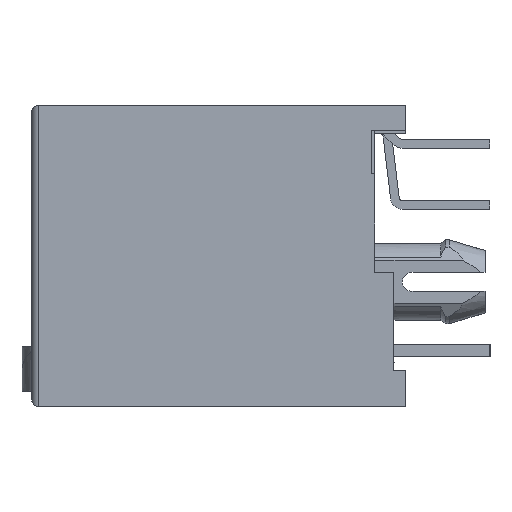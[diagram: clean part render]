
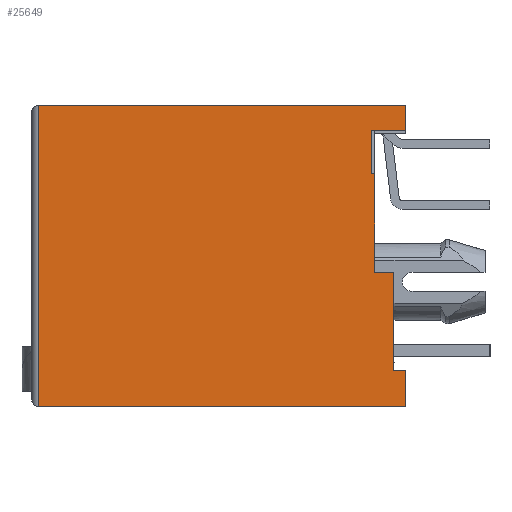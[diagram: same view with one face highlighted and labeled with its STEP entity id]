
A CAD part, left-side view. The second image highlights one B-rep face of the part: STEP entity #25649.
In plain terms, the highlighted planar face has unit normal (-1, 0, 0).
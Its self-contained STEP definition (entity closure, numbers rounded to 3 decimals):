
#753 = CARTESIAN_POINT ( 'NONE',  ( -31.5, -6.35, 5.25 ) ) ;
#794 = B_SPLINE_CURVE_WITH_KNOTS ( 'NONE', 3,
 ( #58635, #41597, #31575, #52711 ),
 .UNSPECIFIED., .F., .F.,
 ( 4, 4 ),
 ( 0., 1. ),
 .UNSPECIFIED. ) ;
#1105 = CARTESIAN_POINT ( 'NONE',  ( -31.5, -7.3, -4.75 ) ) ;
#1653 = FACE_OUTER_BOUND ( 'NONE', #20320, .T. ) ;
#1766 = PLANE ( 'NONE',  #33108 ) ;
#1990 = ORIENTED_EDGE ( 'NONE', *, *, #2348, .F. ) ;
#2241 = CARTESIAN_POINT ( 'NONE',  ( -31.5, 7.806, -6.501 ) ) ;
#2348 = EDGE_CURVE ( 'NONE', #6272, #35705, #45475, .T. ) ;
#3171 = CARTESIAN_POINT ( 'NONE',  ( -31.5, -7.8, 5.95 ) ) ;
#3484 = CARTESIAN_POINT ( 'NONE',  ( -31.5, 7.5, -6.25 ) ) ;
#4537 = CARTESIAN_POINT ( 'NONE',  ( -31.5, -7.317, 5.25 ) ) ;
#4811 = CARTESIAN_POINT ( 'NONE',  ( -31.5, -7.3, -0.65 ) ) ;
#5822 = VERTEX_POINT ( 'NONE', #54290 ) ;
#5999 = CARTESIAN_POINT ( 'NONE',  ( -31.5, -7.3, -0.65 ) ) ;
#6272 = VERTEX_POINT ( 'NONE', #4811 ) ;
#6521 = CARTESIAN_POINT ( 'NONE',  ( -31.5, -7.8, -4.75 ) ) ;
#6751 = CARTESIAN_POINT ( 'NONE',  ( -31.5, -7.633, -4.75 ) ) ;
#7756 = EDGE_CURVE ( 'NONE', #69774, #23498, #36335, .T. ) ;
#8412 = EDGE_CURVE ( 'NONE', #5822, #59870, #36721, .T. ) ;
#8703 = CARTESIAN_POINT ( 'NONE',  ( -31.5, -6.4, 3.45 ) ) ;
#8846 = CARTESIAN_POINT ( 'NONE',  ( -31.5, -7.8, 5.25 ) ) ;
#9797 = EDGE_CURVE ( 'NONE', #43913, #19857, #70163, .T. ) ;
#10039 = CARTESIAN_POINT ( 'NONE',  ( -31.5, -7.8, -6.25 ) ) ;
#10140 = CARTESIAN_POINT ( 'NONE',  ( -31.5, -7.3, -0.65 ) ) ;
#12160 = CARTESIAN_POINT ( 'NONE',  ( -31.5, -7.3, -4.75 ) ) ;
#13658 = CARTESIAN_POINT ( 'NONE',  ( -31.5, -6.5, 3.45 ) ) ;
#14798 = VERTEX_POINT ( 'NONE', #19851 ) ;
#15674 = EDGE_CURVE ( 'NONE', #24459, #54209, #63186, .T. ) ;
#16421 = B_SPLINE_CURVE_WITH_KNOTS ( 'NONE', 3,
 ( #46222, #8703, #41508, #13658 ),
 .UNSPECIFIED., .F., .F.,
 ( 4, 4 ),
 ( 0., 1. ),
 .UNSPECIFIED. ) ;
#17293 = CARTESIAN_POINT ( 'NONE',  ( -31.5, 2.4, 6.3 ) ) ;
#18165 = CARTESIAN_POINT ( 'NONE',  ( -31.5, -7.8, 5.25 ) ) ;
#18745 = B_SPLINE_CURVE_WITH_KNOTS ( 'NONE', 3,
 ( #1105, #39566, #6751, #6521 ),
 .UNSPECIFIED., .F., .F.,
 ( 4, 4 ),
 ( 0., 1. ),
 .UNSPECIFIED. ) ;
#19851 = CARTESIAN_POINT ( 'NONE',  ( -31.5, -6.5, 3.45 ) ) ;
#19857 = VERTEX_POINT ( 'NONE', #50741 ) ;
#20320 = EDGE_LOOP ( 'NONE', ( #28924, #63908, #1990, #67134, #37770, #33921, #66121, #42720, #31346, #48273, #62933, #54552 ) ) ;
#21495 = EDGE_CURVE ( 'NONE', #19857, #14798, #16421, .T. ) ;
#22341 = EDGE_CURVE ( 'NONE', #54209, #23498, #27360, .T. ) ;
#23498 = VERTEX_POINT ( 'NONE', #67031 ) ;
#23927 = CARTESIAN_POINT ( 'NONE',  ( -31.5, -7.8, -4.75 ) ) ;
#24459 = VERTEX_POINT ( 'NONE', #23927 ) ;
#25649 = ADVANCED_FACE ( 'NONE', ( #1653 ), #1766, .F. ) ;
#25745 = CARTESIAN_POINT ( 'NONE',  ( -31.5, -7.8, -4.75 ) ) ;
#27360 = B_SPLINE_CURVE_WITH_KNOTS ( 'NONE', 3,
 ( #43266, #48709, #38516, #59850 ),
 .UNSPECIFIED., .F., .F.,
 ( 4, 4 ),
 ( 0., 1. ),
 .UNSPECIFIED. ) ;
#28924 = ORIENTED_EDGE ( 'NONE', *, *, #15674, .F. ) ;
#29045 = DIRECTION ( 'NONE',  ( 1., 0., 0. ) ) ;
#29296 = CARTESIAN_POINT ( 'NONE',  ( -31.5, -6.35, 4.05 ) ) ;
#30078 = CARTESIAN_POINT ( 'NONE',  ( -31.5, 7.5, 6.3 ) ) ;
#30939 = B_SPLINE_CURVE_WITH_KNOTS ( 'NONE', 3,
 ( #36412, #4537, #47968, #52745 ),
 .UNSPECIFIED., .F., .F.,
 ( 4, 4 ),
 ( 0., 1. ),
 .UNSPECIFIED. ) ;
#31346 = ORIENTED_EDGE ( 'NONE', *, *, #8412, .F. ) ;
#31424 = EDGE_CURVE ( 'NONE', #35705, #24459, #18745, .T. ) ;
#31575 = CARTESIAN_POINT ( 'NONE',  ( -31.5, -6.5, 0.717 ) ) ;
#33108 = AXIS2_PLACEMENT_3D ( 'NONE', #2241, #29045, #45415 ) ;
#33334 = CARTESIAN_POINT ( 'NONE',  ( -31.5, 7.5, 6.3 ) ) ;
#33423 = CARTESIAN_POINT ( 'NONE',  ( -31.5, -2.7, 6.3 ) ) ;
#33921 = ORIENTED_EDGE ( 'NONE', *, *, #21495, .F. ) ;
#34442 = B_SPLINE_CURVE_WITH_KNOTS ( 'NONE', 3,
 ( #47892, #37257, #58598, #10140 ),
 .UNSPECIFIED., .F., .F.,
 ( 4, 4 ),
 ( 0., 1. ),
 .UNSPECIFIED. ) ;
#35705 = VERTEX_POINT ( 'NONE', #12160 ) ;
#36335 = B_SPLINE_CURVE_WITH_KNOTS ( 'NONE', 3,
 ( #30078, #51194, #68269, #3484 ),
 .UNSPECIFIED., .F., .F.,
 ( 4, 4 ),
 ( 0., 1. ),
 .UNSPECIFIED. ) ;
#36412 = CARTESIAN_POINT ( 'NONE',  ( -31.5, -7.8, 5.25 ) ) ;
#36721 = B_SPLINE_CURVE_WITH_KNOTS ( 'NONE', 3,
 ( #62959, #3171, #52290, #8846 ),
 .UNSPECIFIED., .F., .F.,
 ( 4, 4 ),
 ( 0., 1. ),
 .UNSPECIFIED. ) ;
#37158 = CARTESIAN_POINT ( 'NONE',  ( -31.5, -7.8, -5.25 ) ) ;
#37257 = CARTESIAN_POINT ( 'NONE',  ( -31.5, -6.767, -0.65 ) ) ;
#37770 = ORIENTED_EDGE ( 'NONE', *, *, #45168, .F. ) ;
#38516 = CARTESIAN_POINT ( 'NONE',  ( -31.5, 2.4, -6.25 ) ) ;
#38568 = CARTESIAN_POINT ( 'NONE',  ( -31.5, -7.3, -4.75 ) ) ;
#39542 = CARTESIAN_POINT ( 'NONE',  ( -31.5, -6.35, 5.25 ) ) ;
#39566 = CARTESIAN_POINT ( 'NONE',  ( -31.5, -7.467, -4.75 ) ) ;
#40373 = CARTESIAN_POINT ( 'NONE',  ( -31.5, -7.8, -6.25 ) ) ;
#41508 = CARTESIAN_POINT ( 'NONE',  ( -31.5, -6.45, 3.45 ) ) ;
#41597 = CARTESIAN_POINT ( 'NONE',  ( -31.5, -6.5, 2.083 ) ) ;
#42174 = EDGE_CURVE ( 'NONE', #59870, #43913, #30939, .T. ) ;
#42597 = CARTESIAN_POINT ( 'NONE',  ( -31.5, -7.8, -5.75 ) ) ;
#42720 = ORIENTED_EDGE ( 'NONE', *, *, #42174, .F. ) ;
#43266 = CARTESIAN_POINT ( 'NONE',  ( -31.5, -7.8, -6.25 ) ) ;
#43913 = VERTEX_POINT ( 'NONE', #753 ) ;
#44025 = CARTESIAN_POINT ( 'NONE',  ( -31.5, -7.3, -2.017 ) ) ;
#45168 = EDGE_CURVE ( 'NONE', #14798, #53177, #794, .T. ) ;
#45415 = DIRECTION ( 'NONE',  ( 0., 0., 1. ) ) ;
#45475 = B_SPLINE_CURVE_WITH_KNOTS ( 'NONE', 3,
 ( #5999, #44025, #59679, #38568 ),
 .UNSPECIFIED., .F., .F.,
 ( 4, 4 ),
 ( 0., 1. ),
 .UNSPECIFIED. ) ;
#46222 = CARTESIAN_POINT ( 'NONE',  ( -31.5, -6.35, 3.45 ) ) ;
#46811 = EDGE_CURVE ( 'NONE', #5822, #69774, #50345, .T. ) ;
#47892 = CARTESIAN_POINT ( 'NONE',  ( -31.5, -6.5, -0.65 ) ) ;
#47968 = CARTESIAN_POINT ( 'NONE',  ( -31.5, -6.833, 5.25 ) ) ;
#48273 = ORIENTED_EDGE ( 'NONE', *, *, #46811, .T. ) ;
#48709 = CARTESIAN_POINT ( 'NONE',  ( -31.5, -2.7, -6.25 ) ) ;
#50345 = B_SPLINE_CURVE_WITH_KNOTS ( 'NONE', 3,
 ( #60474, #33423, #17293, #65718 ),
 .UNSPECIFIED., .F., .F.,
 ( 4, 4 ),
 ( 0., 1. ),
 .UNSPECIFIED. ) ;
#50741 = CARTESIAN_POINT ( 'NONE',  ( -31.5, -6.35, 3.45 ) ) ;
#51194 = CARTESIAN_POINT ( 'NONE',  ( -31.5, 7.5, 2.117 ) ) ;
#52290 = CARTESIAN_POINT ( 'NONE',  ( -31.5, -7.8, 5.6 ) ) ;
#52711 = CARTESIAN_POINT ( 'NONE',  ( -31.5, -6.5, -0.65 ) ) ;
#52745 = CARTESIAN_POINT ( 'NONE',  ( -31.5, -6.35, 5.25 ) ) ;
#53177 = VERTEX_POINT ( 'NONE', #68028 ) ;
#54209 = VERTEX_POINT ( 'NONE', #40373 ) ;
#54290 = CARTESIAN_POINT ( 'NONE',  ( -31.5, -7.8, 6.3 ) ) ;
#54552 = ORIENTED_EDGE ( 'NONE', *, *, #22341, .F. ) ;
#55433 = CARTESIAN_POINT ( 'NONE',  ( -31.5, -6.35, 3.45 ) ) ;
#58598 = CARTESIAN_POINT ( 'NONE',  ( -31.5, -7.033, -0.65 ) ) ;
#58635 = CARTESIAN_POINT ( 'NONE',  ( -31.5, -6.5, 3.45 ) ) ;
#59679 = CARTESIAN_POINT ( 'NONE',  ( -31.5, -7.3, -3.383 ) ) ;
#59850 = CARTESIAN_POINT ( 'NONE',  ( -31.5, 7.5, -6.25 ) ) ;
#59870 = VERTEX_POINT ( 'NONE', #18165 ) ;
#60474 = CARTESIAN_POINT ( 'NONE',  ( -31.5, -7.8, 6.3 ) ) ;
#60863 = CARTESIAN_POINT ( 'NONE',  ( -31.5, -6.35, 4.65 ) ) ;
#62933 = ORIENTED_EDGE ( 'NONE', *, *, #7756, .T. ) ;
#62959 = CARTESIAN_POINT ( 'NONE',  ( -31.5, -7.8, 6.3 ) ) ;
#63186 = B_SPLINE_CURVE_WITH_KNOTS ( 'NONE', 3,
 ( #25745, #37158, #42597, #10039 ),
 .UNSPECIFIED., .F., .F.,
 ( 4, 4 ),
 ( 0., 1. ),
 .UNSPECIFIED. ) ;
#63908 = ORIENTED_EDGE ( 'NONE', *, *, #31424, .F. ) ;
#65718 = CARTESIAN_POINT ( 'NONE',  ( -31.5, 7.5, 6.3 ) ) ;
#66121 = ORIENTED_EDGE ( 'NONE', *, *, #9797, .F. ) ;
#67031 = CARTESIAN_POINT ( 'NONE',  ( -31.5, 7.5, -6.25 ) ) ;
#67134 = ORIENTED_EDGE ( 'NONE', *, *, #67436, .F. ) ;
#67436 = EDGE_CURVE ( 'NONE', #53177, #6272, #34442, .T. ) ;
#68028 = CARTESIAN_POINT ( 'NONE',  ( -31.5, -6.5, -0.65 ) ) ;
#68269 = CARTESIAN_POINT ( 'NONE',  ( -31.5, 7.5, -2.067 ) ) ;
#69774 = VERTEX_POINT ( 'NONE', #33334 ) ;
#70163 = B_SPLINE_CURVE_WITH_KNOTS ( 'NONE', 3,
 ( #39542, #60863, #29296, #55433 ),
 .UNSPECIFIED., .F., .F.,
 ( 4, 4 ),
 ( 0., 1. ),
 .UNSPECIFIED. ) ;
